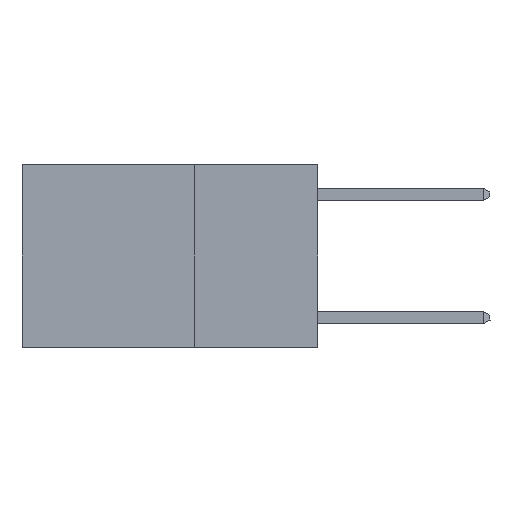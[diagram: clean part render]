
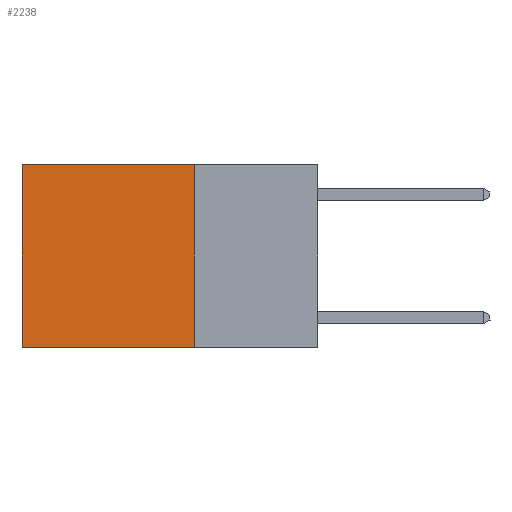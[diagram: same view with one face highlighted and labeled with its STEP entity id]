
A CAD part, left-side view. The second image highlights one B-rep face of the part: STEP entity #2238.
In plain terms, the highlighted planar face has unit normal (-1, 0, 0).
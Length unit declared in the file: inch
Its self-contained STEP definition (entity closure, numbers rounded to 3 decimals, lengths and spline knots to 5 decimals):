
#848 = LINE ( 'NONE', #22374, #17078 ) ;
#1612 = CARTESIAN_POINT ( 'NONE',  ( 0.2625, 0.6, -0.37 ) ) ;
#1712 = EDGE_CURVE ( 'NONE', #8008, #5520, #8112, .T. ) ;
#2238 = ADVANCED_FACE ( 'NONE', ( #22645 ), #3405, .F. ) ;
#2411 = VECTOR ( 'NONE', #20740, 39.37008 ) ;
#2800 = AXIS2_PLACEMENT_3D ( 'NONE', #7620, #18132, #5574 ) ;
#3405 = PLANE ( 'NONE',  #2800 ) ;
#5520 = VERTEX_POINT ( 'NONE', #1612 ) ;
#5574 = DIRECTION ( 'NONE',  ( 0., 0., -1. ) ) ;
#5921 = CARTESIAN_POINT ( 'NONE',  ( 0.2625, 0.25, 0. ) ) ;
#7620 = CARTESIAN_POINT ( 'NONE',  ( 0.2625, 0.25, 0. ) ) ;
#8008 = VERTEX_POINT ( 'NONE', #8819 ) ;
#8112 = LINE ( 'NONE', #18603, #2411 ) ;
#8247 = CARTESIAN_POINT ( 'NONE',  ( 0.2625, 0.25, 0. ) ) ;
#8819 = CARTESIAN_POINT ( 'NONE',  ( 0.2625, 0.25, -0.37 ) ) ;
#8951 = EDGE_CURVE ( 'NONE', #14103, #19084, #26644, .T. ) ;
#8958 = LINE ( 'NONE', #8247, #24766 ) ;
#9023 = EDGE_CURVE ( 'NONE', #14103, #8008, #8958, .T. ) ;
#11157 = EDGE_LOOP ( 'NONE', ( #23261, #14798, #15130, #16042 ) ) ;
#14103 = VERTEX_POINT ( 'NONE', #24069 ) ;
#14798 = ORIENTED_EDGE ( 'NONE', *, *, #1712, .F. ) ;
#15130 = ORIENTED_EDGE ( 'NONE', *, *, #9023, .F. ) ;
#16042 = ORIENTED_EDGE ( 'NONE', *, *, #8951, .T. ) ;
#16254 = DIRECTION ( 'NONE',  ( 0., 0., -1. ) ) ;
#17078 = VECTOR ( 'NONE', #16254, 39.37008 ) ;
#18132 = DIRECTION ( 'NONE',  ( 1., 0., 0. ) ) ;
#18603 = CARTESIAN_POINT ( 'NONE',  ( 0.2625, 0.25, -0.37 ) ) ;
#18635 = DIRECTION ( 'NONE',  ( 0., 0., -1. ) ) ;
#19084 = VERTEX_POINT ( 'NONE', #23814 ) ;
#20510 = DIRECTION ( 'NONE',  ( 0., 1., 0. ) ) ;
#20740 = DIRECTION ( 'NONE',  ( 0., 1., 0. ) ) ;
#21287 = VECTOR ( 'NONE', #20510, 39.37008 ) ;
#22374 = CARTESIAN_POINT ( 'NONE',  ( 0.2625, 0.6, 0. ) ) ;
#22645 = FACE_OUTER_BOUND ( 'NONE', #11157, .T. ) ;
#23261 = ORIENTED_EDGE ( 'NONE', *, *, #26043, .T. ) ;
#23814 = CARTESIAN_POINT ( 'NONE',  ( 0.2625, 0.6, 0. ) ) ;
#24069 = CARTESIAN_POINT ( 'NONE',  ( 0.2625, 0.25, 0. ) ) ;
#24766 = VECTOR ( 'NONE', #18635, 39.37008 ) ;
#26043 = EDGE_CURVE ( 'NONE', #19084, #5520, #848, .T. ) ;
#26644 = LINE ( 'NONE', #5921, #21287 ) ;
